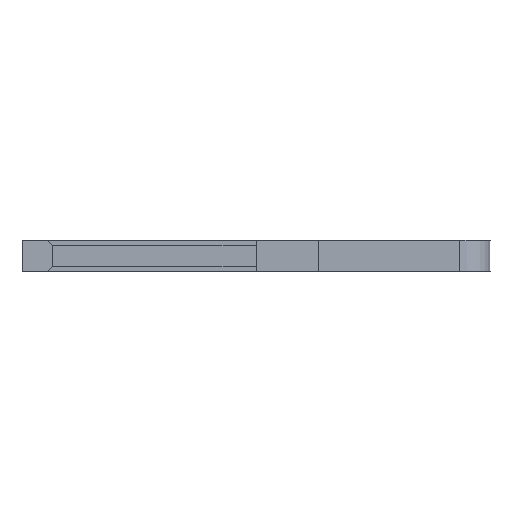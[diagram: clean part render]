
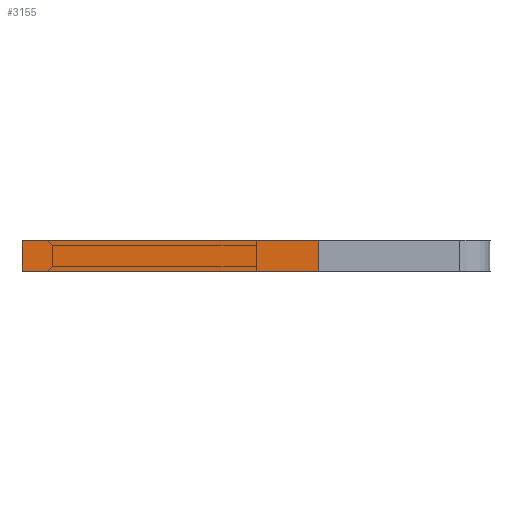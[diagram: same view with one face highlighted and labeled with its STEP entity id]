
A CAD part, left-side view. The second image highlights one B-rep face of the part: STEP entity #3155.
In plain terms, the highlighted face is planar.
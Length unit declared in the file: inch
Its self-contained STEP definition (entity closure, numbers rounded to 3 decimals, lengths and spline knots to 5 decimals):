
#16 = VECTOR ( 'NONE', #1729, 39.37008 ) ;
#94 = CARTESIAN_POINT ( 'NONE',  ( 0.01, 0.15, -0.04 ) ) ;
#178 = EDGE_CURVE ( 'NONE', #4392, #2943, #3505, .T. ) ;
#522 = CARTESIAN_POINT ( 'NONE',  ( 0.01, 0.15, -0.04 ) ) ;
#804 = DIRECTION ( 'NONE',  ( 1., 0., 0. ) ) ;
#868 = CARTESIAN_POINT ( 'NONE',  ( 0.01, -0.04, -0.04 ) ) ;
#1155 = FACE_OUTER_BOUND ( 'NONE', #4389, .T. ) ;
#1157 = AXIS2_PLACEMENT_3D ( 'NONE', #94, #4088, #804 ) ;
#1187 = CARTESIAN_POINT ( 'NONE',  ( 0.01, 0.15, -0.04 ) ) ;
#1578 = DIRECTION ( 'NONE',  ( 0., 1., 0. ) ) ;
#1729 = DIRECTION ( 'NONE',  ( -1., 0., 0. ) ) ;
#1850 = VECTOR ( 'NONE', #3813, 39.37008 ) ;
#1868 = EDGE_CURVE ( 'NONE', #2774, #4196, #4578, .T. ) ;
#1890 = CARTESIAN_POINT ( 'NONE',  ( 0.01, 0.15, -0.04 ) ) ;
#1892 = EDGE_CURVE ( 'NONE', #2943, #4196, #2658, .T. ) ;
#2138 = ORIENTED_EDGE ( 'NONE', *, *, #1892, .T. ) ;
#2481 = ORIENTED_EDGE ( 'NONE', *, *, #178, .T. ) ;
#2656 = PLANE ( 'NONE',  #1157 ) ;
#2658 = LINE ( 'NONE', #2728, #4297 ) ;
#2728 = CARTESIAN_POINT ( 'NONE',  ( -0.01, 0.15, -0.04 ) ) ;
#2774 = VERTEX_POINT ( 'NONE', #1890 ) ;
#2943 = VERTEX_POINT ( 'NONE', #3713 ) ;
#3155 = ADVANCED_FACE ( 'NONE', ( #1155 ), #2656, .F. ) ;
#3270 = ORIENTED_EDGE ( 'NONE', *, *, #1868, .F. ) ;
#3344 = ORIENTED_EDGE ( 'NONE', *, *, #4507, .F. ) ;
#3382 = DIRECTION ( 'NONE',  ( -1., 0., 0. ) ) ;
#3505 = LINE ( 'NONE', #3890, #16 ) ;
#3630 = VECTOR ( 'NONE', #3382, 39.37008 ) ;
#3713 = CARTESIAN_POINT ( 'NONE',  ( -0.01, -0.04, -0.04 ) ) ;
#3813 = DIRECTION ( 'NONE',  ( 0., 1., 0. ) ) ;
#3890 = CARTESIAN_POINT ( 'NONE',  ( 0.01, -0.04, -0.04 ) ) ;
#3963 = LINE ( 'NONE', #1187, #1850 ) ;
#4088 = DIRECTION ( 'NONE',  ( 0., 0., 1. ) ) ;
#4196 = VERTEX_POINT ( 'NONE', #4539 ) ;
#4297 = VECTOR ( 'NONE', #1578, 39.37008 ) ;
#4389 = EDGE_LOOP ( 'NONE', ( #2138, #3270, #3344, #2481 ) ) ;
#4392 = VERTEX_POINT ( 'NONE', #868 ) ;
#4507 = EDGE_CURVE ( 'NONE', #4392, #2774, #3963, .T. ) ;
#4539 = CARTESIAN_POINT ( 'NONE',  ( -0.01, 0.15, -0.04 ) ) ;
#4578 = LINE ( 'NONE', #522, #3630 ) ;
